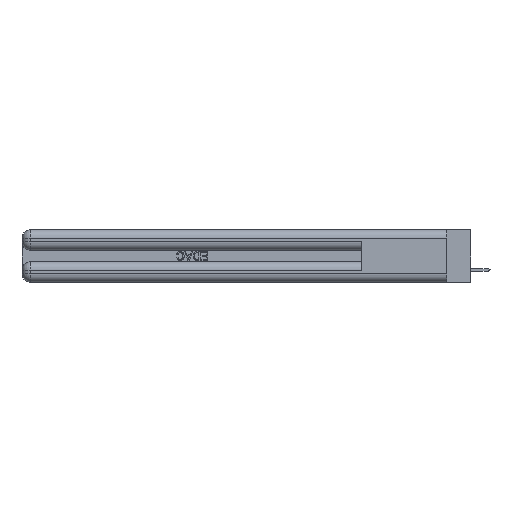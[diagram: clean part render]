
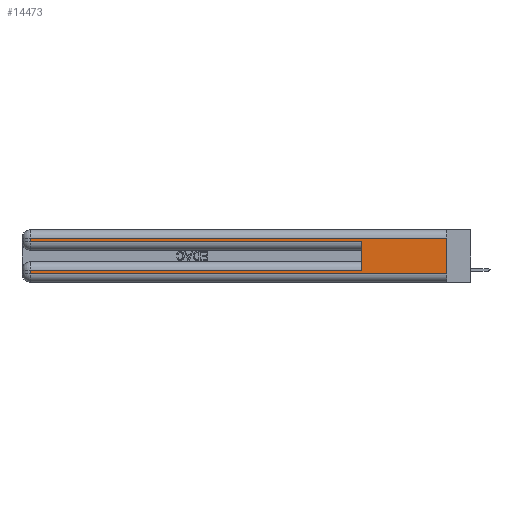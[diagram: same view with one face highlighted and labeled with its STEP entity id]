
A CAD part, left-side view. The second image highlights one B-rep face of the part: STEP entity #14473.
In plain terms, the highlighted planar face has unit normal (-1, 0, 0).
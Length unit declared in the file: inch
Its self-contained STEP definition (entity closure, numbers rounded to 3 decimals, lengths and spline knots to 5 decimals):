
#1118 = EDGE_CURVE ( 'NONE', #22440, #1861, #24823, .T. ) ;
#1861 = VERTEX_POINT ( 'NONE', #13203 ) ;
#2053 = LINE ( 'NONE', #31984, #20341 ) ;
#2338 = LINE ( 'NONE', #13430, #21780 ) ;
#2718 = VERTEX_POINT ( 'NONE', #12654 ) ;
#2753 = DIRECTION ( 'NONE',  ( 0., 0., -1. ) ) ;
#3114 = CARTESIAN_POINT ( 'NONE',  ( 0., 2.94, 0.085 ) ) ;
#4090 = EDGE_CURVE ( 'NONE', #2718, #1861, #24376, .T. ) ;
#4962 = DIRECTION ( 'NONE',  ( 0., 0., -1. ) ) ;
#5149 = ORIENTED_EDGE ( 'NONE', *, *, #1118, .T. ) ;
#5165 = DIRECTION ( 'NONE',  ( 0., 0., -1. ) ) ;
#5371 = PLANE ( 'NONE',  #34562 ) ;
#5911 = VERTEX_POINT ( 'NONE', #20669 ) ;
#6404 = ORIENTED_EDGE ( 'NONE', *, *, #4090, .F. ) ;
#6589 = EDGE_CURVE ( 'NONE', #5911, #27238, #19015, .T. ) ;
#8183 = CARTESIAN_POINT ( 'NONE',  ( 0., 0., 0.06 ) ) ;
#10052 = LINE ( 'NONE', #19373, #30469 ) ;
#10098 = ORIENTED_EDGE ( 'NONE', *, *, #36808, .F. ) ;
#12018 = FACE_OUTER_BOUND ( 'NONE', #39611, .T. ) ;
#12359 = DIRECTION ( 'NONE',  ( 0., 1., 0. ) ) ;
#12654 = CARTESIAN_POINT ( 'NONE',  ( 0., 0., 0.31 ) ) ;
#13082 = LINE ( 'NONE', #40131, #43092 ) ;
#13093 = VECTOR ( 'NONE', #21705, 39.37008 ) ;
#13203 = CARTESIAN_POINT ( 'NONE',  ( 0., 0., 0.06 ) ) ;
#13430 = CARTESIAN_POINT ( 'NONE',  ( 0., 0., 0.31 ) ) ;
#13981 = DIRECTION ( 'NONE',  ( 0., 0., -1. ) ) ;
#14473 = ADVANCED_FACE ( 'NONE', ( #12018 ), #5371, .F. ) ;
#14503 = VERTEX_POINT ( 'NONE', #39273 ) ;
#15079 = EDGE_CURVE ( 'NONE', #33083, #14503, #13082, .T. ) ;
#17362 = DIRECTION ( 'NONE',  ( 0., 0., 1. ) ) ;
#19015 = LINE ( 'NONE', #32538, #26078 ) ;
#19373 = CARTESIAN_POINT ( 'NONE',  ( 0., 2.94, 0.37 ) ) ;
#20341 = VECTOR ( 'NONE', #4962, 39.37008 ) ;
#20669 = CARTESIAN_POINT ( 'NONE',  ( 0., 0.6, 0.085 ) ) ;
#21705 = DIRECTION ( 'NONE',  ( 0., -1., 0. ) ) ;
#21780 = VECTOR ( 'NONE', #29613, 39.37008 ) ;
#22440 = VERTEX_POINT ( 'NONE', #42349 ) ;
#22647 = CARTESIAN_POINT ( 'NONE',  ( 0., 0., 0.37 ) ) ;
#24376 = LINE ( 'NONE', #41444, #34513 ) ;
#24390 = ORIENTED_EDGE ( 'NONE', *, *, #6589, .T. ) ;
#24823 = LINE ( 'NONE', #8183, #13093 ) ;
#26078 = VECTOR ( 'NONE', #12359, 39.37008 ) ;
#26216 = CARTESIAN_POINT ( 'NONE',  ( 0., 2.94, 0.285 ) ) ;
#26217 = VECTOR ( 'NONE', #17362, 39.37008 ) ;
#26947 = CARTESIAN_POINT ( 'NONE',  ( 0., 2.94, 0.31 ) ) ;
#27128 = LINE ( 'NONE', #34218, #26217 ) ;
#27238 = VERTEX_POINT ( 'NONE', #3114 ) ;
#28844 = ORIENTED_EDGE ( 'NONE', *, *, #36676, .T. ) ;
#29613 = DIRECTION ( 'NONE',  ( 0., 1., 0. ) ) ;
#30469 = VECTOR ( 'NONE', #2753, 39.37008 ) ;
#31984 = CARTESIAN_POINT ( 'NONE',  ( 0., 2.94, 0.37 ) ) ;
#32415 = DIRECTION ( 'NONE',  ( 1., 0., 0. ) ) ;
#32538 = CARTESIAN_POINT ( 'NONE',  ( 0., 0., 0.085 ) ) ;
#32700 = ORIENTED_EDGE ( 'NONE', *, *, #32896, .T. ) ;
#32896 = EDGE_CURVE ( 'NONE', #27238, #22440, #2053, .T. ) ;
#33031 = DIRECTION ( 'NONE',  ( 0., -1., 0. ) ) ;
#33083 = VERTEX_POINT ( 'NONE', #26216 ) ;
#33858 = VERTEX_POINT ( 'NONE', #26947 ) ;
#33877 = EDGE_CURVE ( 'NONE', #2718, #33858, #2338, .T. ) ;
#34218 = CARTESIAN_POINT ( 'NONE',  ( 0., 0.6, 0.145 ) ) ;
#34513 = VECTOR ( 'NONE', #13981, 39.37008 ) ;
#34562 = AXIS2_PLACEMENT_3D ( 'NONE', #22647, #32415, #5165 ) ;
#36676 = EDGE_CURVE ( 'NONE', #33858, #33083, #10052, .T. ) ;
#36808 = EDGE_CURVE ( 'NONE', #5911, #14503, #27128, .T. ) ;
#39273 = CARTESIAN_POINT ( 'NONE',  ( 0., 0.6, 0.285 ) ) ;
#39611 = EDGE_LOOP ( 'NONE', ( #6404, #42495, #28844, #41590, #10098, #24390, #32700, #5149 ) ) ;
#40131 = CARTESIAN_POINT ( 'NONE',  ( 0., 0., 0.285 ) ) ;
#41444 = CARTESIAN_POINT ( 'NONE',  ( 0., 0., 0.37 ) ) ;
#41590 = ORIENTED_EDGE ( 'NONE', *, *, #15079, .T. ) ;
#42349 = CARTESIAN_POINT ( 'NONE',  ( 0., 2.94, 0.06 ) ) ;
#42495 = ORIENTED_EDGE ( 'NONE', *, *, #33877, .T. ) ;
#43092 = VECTOR ( 'NONE', #33031, 39.37008 ) ;
